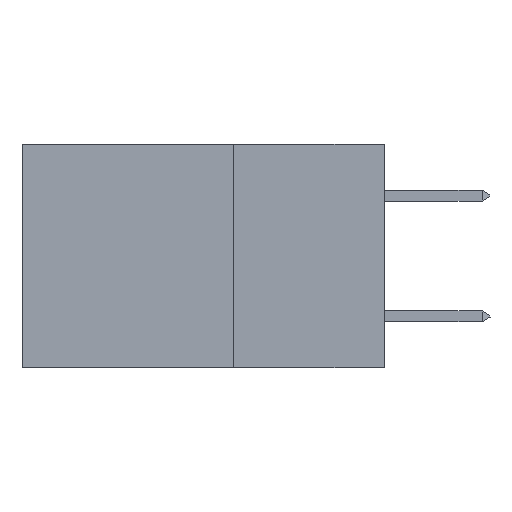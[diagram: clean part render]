
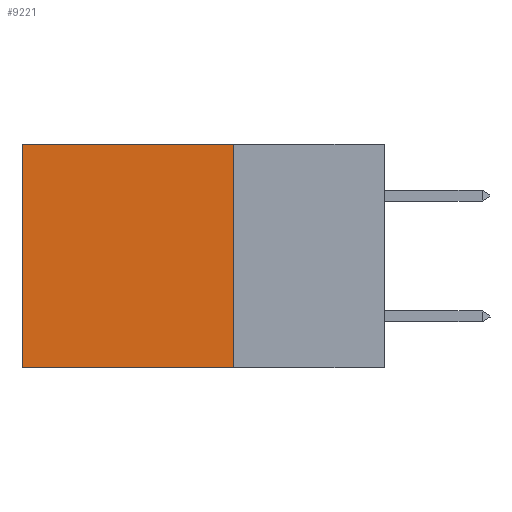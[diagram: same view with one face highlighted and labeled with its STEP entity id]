
A CAD part, left-side view. The second image highlights one B-rep face of the part: STEP entity #9221.
In plain terms, the highlighted planar face has unit normal (-1, 0, 0).
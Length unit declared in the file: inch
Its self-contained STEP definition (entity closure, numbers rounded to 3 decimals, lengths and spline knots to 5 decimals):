
#573 = VERTEX_POINT ( 'NONE', #29408 ) ;
#2089 = FACE_OUTER_BOUND ( 'NONE', #8765, .T. ) ;
#3015 = LINE ( 'NONE', #18608, #17799 ) ;
#3585 = LINE ( 'NONE', #34873, #18383 ) ;
#4556 = ORIENTED_EDGE ( 'NONE', *, *, #32986, .T. ) ;
#5626 = CARTESIAN_POINT ( 'NONE',  ( 0.2875, 0.25, -0.37 ) ) ;
#5854 = VERTEX_POINT ( 'NONE', #30934 ) ;
#5987 = ORIENTED_EDGE ( 'NONE', *, *, #25758, .F. ) ;
#8414 = CARTESIAN_POINT ( 'NONE',  ( 0.2875, 0.6, -0.37 ) ) ;
#8765 = EDGE_LOOP ( 'NONE', ( #4556, #5987, #33695, #16164 ) ) ;
#9221 = ADVANCED_FACE ( 'NONE', ( #2089 ), #13782, .F. ) ;
#9930 = AXIS2_PLACEMENT_3D ( 'NONE', #32696, #35424, #19245 ) ;
#12560 = EDGE_CURVE ( 'NONE', #29365, #5854, #15159, .T. ) ;
#13731 = DIRECTION ( 'NONE',  ( 0., 0., -1. ) ) ;
#13782 = PLANE ( 'NONE',  #9930 ) ;
#15159 = LINE ( 'NONE', #21933, #23221 ) ;
#16164 = ORIENTED_EDGE ( 'NONE', *, *, #24227, .T. ) ;
#17799 = VECTOR ( 'NONE', #34787, 39.37008 ) ;
#18383 = VECTOR ( 'NONE', #18697, 39.37008 ) ;
#18608 = CARTESIAN_POINT ( 'NONE',  ( 0.2875, 0.6, 0. ) ) ;
#18687 = VECTOR ( 'NONE', #27560, 39.37008 ) ;
#18697 = DIRECTION ( 'NONE',  ( 0., 1., 0. ) ) ;
#19245 = DIRECTION ( 'NONE',  ( 0., 0., -1. ) ) ;
#20379 = LINE ( 'NONE', #5626, #18687 ) ;
#21933 = CARTESIAN_POINT ( 'NONE',  ( 0.2875, 0.25, 0. ) ) ;
#23221 = VECTOR ( 'NONE', #13731, 39.37008 ) ;
#24227 = EDGE_CURVE ( 'NONE', #29365, #573, #3585, .T. ) ;
#25758 = EDGE_CURVE ( 'NONE', #5854, #28679, #20379, .T. ) ;
#27560 = DIRECTION ( 'NONE',  ( 0., 1., 0. ) ) ;
#28679 = VERTEX_POINT ( 'NONE', #8414 ) ;
#29365 = VERTEX_POINT ( 'NONE', #30298 ) ;
#29408 = CARTESIAN_POINT ( 'NONE',  ( 0.2875, 0.6, 0. ) ) ;
#30298 = CARTESIAN_POINT ( 'NONE',  ( 0.2875, 0.25, 0. ) ) ;
#30934 = CARTESIAN_POINT ( 'NONE',  ( 0.2875, 0.25, -0.37 ) ) ;
#32696 = CARTESIAN_POINT ( 'NONE',  ( 0.2875, 0.25, 0. ) ) ;
#32986 = EDGE_CURVE ( 'NONE', #573, #28679, #3015, .T. ) ;
#33695 = ORIENTED_EDGE ( 'NONE', *, *, #12560, .F. ) ;
#34787 = DIRECTION ( 'NONE',  ( 0., 0., -1. ) ) ;
#34873 = CARTESIAN_POINT ( 'NONE',  ( 0.2875, 0.25, 0. ) ) ;
#35424 = DIRECTION ( 'NONE',  ( 1., 0., 0. ) ) ;
